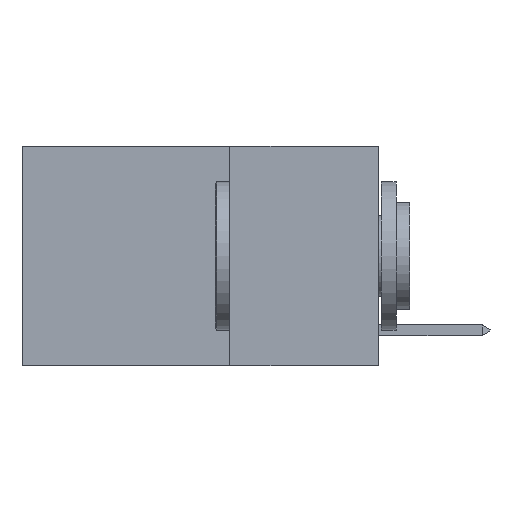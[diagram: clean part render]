
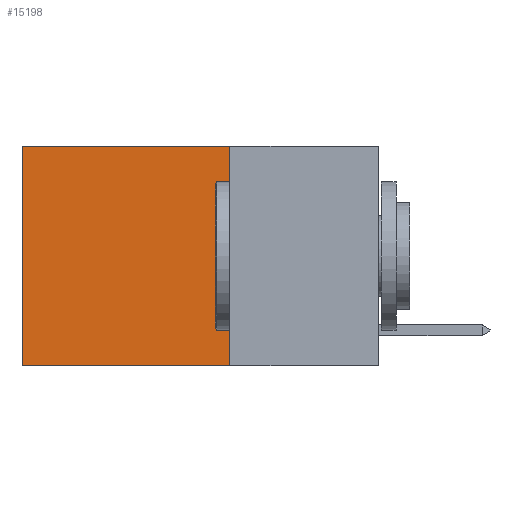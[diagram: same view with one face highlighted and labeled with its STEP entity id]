
A CAD part, left-side view. The second image highlights one B-rep face of the part: STEP entity #15198.
In plain terms, the highlighted planar face has unit normal (-1, 0, 0).
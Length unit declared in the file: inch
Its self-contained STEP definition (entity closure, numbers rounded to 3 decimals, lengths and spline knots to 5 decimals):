
#447 = VERTEX_POINT ( 'NONE', #6492 ) ;
#901 = CARTESIAN_POINT ( 'NONE',  ( 0.2625, 0.25, 0. ) ) ;
#1239 = LINE ( 'NONE', #18004, #9294 ) ;
#2208 = ORIENTED_EDGE ( 'NONE', *, *, #24181, .F. ) ;
#2256 = CARTESIAN_POINT ( 'NONE',  ( 0.2625, 0.25, 0. ) ) ;
#2657 = LINE ( 'NONE', #901, #6374 ) ;
#3720 = VECTOR ( 'NONE', #14446, 39.37008 ) ;
#4059 = DIRECTION ( 'NONE',  ( 1., 0., 0. ) ) ;
#4070 = VERTEX_POINT ( 'NONE', #2256 ) ;
#5218 = CARTESIAN_POINT ( 'NONE',  ( 0.2625, 0.6, 0. ) ) ;
#5675 = EDGE_LOOP ( 'NONE', ( #20069, #23593, #2208, #13422 ) ) ;
#5909 = FACE_OUTER_BOUND ( 'NONE', #5675, .T. ) ;
#6289 = CARTESIAN_POINT ( 'NONE',  ( 0.2625, 0.6, -0.37 ) ) ;
#6374 = VECTOR ( 'NONE', #23826, 39.37008 ) ;
#6492 = CARTESIAN_POINT ( 'NONE',  ( 0.2625, 0.6, 0. ) ) ;
#6955 = LINE ( 'NONE', #14575, #3720 ) ;
#7740 = EDGE_CURVE ( 'NONE', #4070, #447, #6955, .T. ) ;
#9294 = VECTOR ( 'NONE', #21492, 39.37008 ) ;
#9668 = DIRECTION ( 'NONE',  ( 0., 0., -1. ) ) ;
#10820 = LINE ( 'NONE', #5218, #20081 ) ;
#13371 = CARTESIAN_POINT ( 'NONE',  ( 0.2625, 0.25, 0. ) ) ;
#13422 = ORIENTED_EDGE ( 'NONE', *, *, #7740, .T. ) ;
#14446 = DIRECTION ( 'NONE',  ( 0., 1., 0. ) ) ;
#14516 = AXIS2_PLACEMENT_3D ( 'NONE', #13371, #4059, #9668 ) ;
#14575 = CARTESIAN_POINT ( 'NONE',  ( 0.2625, 0.25, 0. ) ) ;
#15198 = ADVANCED_FACE ( 'NONE', ( #5909 ), #19121, .F. ) ;
#16376 = CARTESIAN_POINT ( 'NONE',  ( 0.2625, 0.25, -0.37 ) ) ;
#17302 = EDGE_CURVE ( 'NONE', #20565, #21283, #1239, .T. ) ;
#18004 = CARTESIAN_POINT ( 'NONE',  ( 0.2625, 0.25, -0.37 ) ) ;
#18291 = DIRECTION ( 'NONE',  ( 0., 0., -1. ) ) ;
#19121 = PLANE ( 'NONE',  #14516 ) ;
#19274 = EDGE_CURVE ( 'NONE', #447, #21283, #10820, .T. ) ;
#20069 = ORIENTED_EDGE ( 'NONE', *, *, #19274, .T. ) ;
#20081 = VECTOR ( 'NONE', #18291, 39.37008 ) ;
#20565 = VERTEX_POINT ( 'NONE', #16376 ) ;
#21283 = VERTEX_POINT ( 'NONE', #6289 ) ;
#21492 = DIRECTION ( 'NONE',  ( 0., 1., 0. ) ) ;
#23593 = ORIENTED_EDGE ( 'NONE', *, *, #17302, .F. ) ;
#23826 = DIRECTION ( 'NONE',  ( 0., 0., -1. ) ) ;
#24181 = EDGE_CURVE ( 'NONE', #4070, #20565, #2657, .T. ) ;
